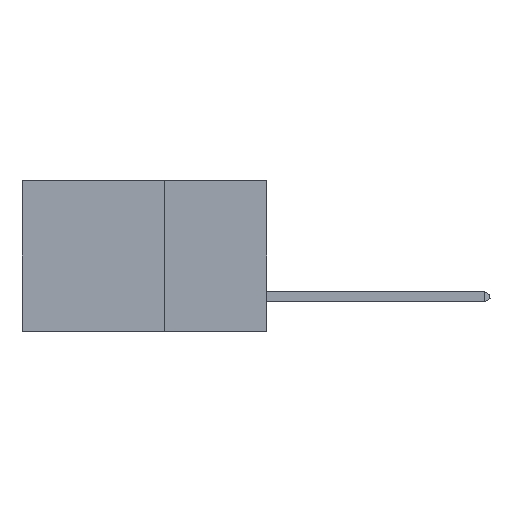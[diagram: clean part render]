
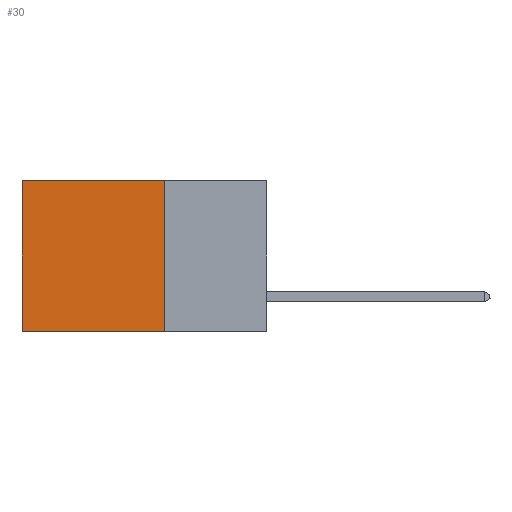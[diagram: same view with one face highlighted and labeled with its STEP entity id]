
A CAD part, left-side view. The second image highlights one B-rep face of the part: STEP entity #30.
In plain terms, the highlighted planar face has unit normal (-1, 0, 0).
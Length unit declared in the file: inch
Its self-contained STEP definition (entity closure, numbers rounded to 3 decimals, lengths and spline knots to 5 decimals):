
#30 = ADVANCED_FACE ( 'NONE', ( #5145 ), #9053, .F. ) ;
#215 = CARTESIAN_POINT ( 'NONE',  ( 0.2875, 0.25, 0. ) ) ;
#1098 = ORIENTED_EDGE ( 'NONE', *, *, #15076, .F. ) ;
#1425 = DIRECTION ( 'NONE',  ( 0., 1., 0. ) ) ;
#1981 = CARTESIAN_POINT ( 'NONE',  ( 0.2875, 0.25, 0. ) ) ;
#2058 = CARTESIAN_POINT ( 'NONE',  ( 0.2875, 0.6, -0.37 ) ) ;
#3173 = LINE ( 'NONE', #16463, #19508 ) ;
#4438 = EDGE_LOOP ( 'NONE', ( #9976, #1098, #5991, #5508 ) ) ;
#4451 = VECTOR ( 'NONE', #1425, 39.37008 ) ;
#4777 = CARTESIAN_POINT ( 'NONE',  ( 0.2875, 0.6, 0. ) ) ;
#4921 = EDGE_CURVE ( 'NONE', #17509, #5551, #3173, .T. ) ;
#5018 = DIRECTION ( 'NONE',  ( 0., 0., -1. ) ) ;
#5145 = FACE_OUTER_BOUND ( 'NONE', #4438, .T. ) ;
#5441 = DIRECTION ( 'NONE',  ( 0., 0., -1. ) ) ;
#5508 = ORIENTED_EDGE ( 'NONE', *, *, #19231, .T. ) ;
#5551 = VERTEX_POINT ( 'NONE', #2058 ) ;
#5991 = ORIENTED_EDGE ( 'NONE', *, *, #6478, .F. ) ;
#6077 = VERTEX_POINT ( 'NONE', #16061 ) ;
#6083 = VECTOR ( 'NONE', #5018, 39.37008 ) ;
#6478 = EDGE_CURVE ( 'NONE', #6077, #19684, #18715, .T. ) ;
#6713 = AXIS2_PLACEMENT_3D ( 'NONE', #9632, #6807, #19485 ) ;
#6807 = DIRECTION ( 'NONE',  ( 1., 0., 0. ) ) ;
#9053 = PLANE ( 'NONE',  #6713 ) ;
#9632 = CARTESIAN_POINT ( 'NONE',  ( 0.2875, 0.25, 0. ) ) ;
#9976 = ORIENTED_EDGE ( 'NONE', *, *, #4921, .T. ) ;
#10850 = CARTESIAN_POINT ( 'NONE',  ( 0.2875, 0.25, -0.37 ) ) ;
#12810 = LINE ( 'NONE', #20212, #4451 ) ;
#12991 = DIRECTION ( 'NONE',  ( 0., 1., 0. ) ) ;
#14427 = VECTOR ( 'NONE', #12991, 39.37008 ) ;
#15076 = EDGE_CURVE ( 'NONE', #19684, #5551, #12810, .T. ) ;
#16061 = CARTESIAN_POINT ( 'NONE',  ( 0.2875, 0.25, 0. ) ) ;
#16463 = CARTESIAN_POINT ( 'NONE',  ( 0.2875, 0.6, 0. ) ) ;
#17509 = VERTEX_POINT ( 'NONE', #4777 ) ;
#17679 = LINE ( 'NONE', #215, #14427 ) ;
#18715 = LINE ( 'NONE', #1981, #6083 ) ;
#19231 = EDGE_CURVE ( 'NONE', #6077, #17509, #17679, .T. ) ;
#19485 = DIRECTION ( 'NONE',  ( 0., 0., -1. ) ) ;
#19508 = VECTOR ( 'NONE', #5441, 39.37008 ) ;
#19684 = VERTEX_POINT ( 'NONE', #10850 ) ;
#20212 = CARTESIAN_POINT ( 'NONE',  ( 0.2875, 0.25, -0.37 ) ) ;
